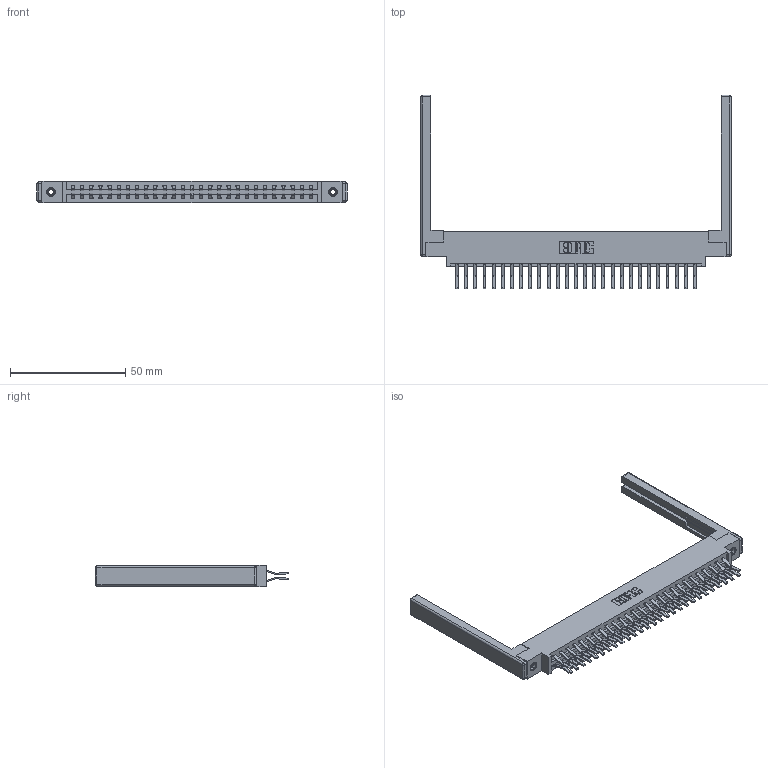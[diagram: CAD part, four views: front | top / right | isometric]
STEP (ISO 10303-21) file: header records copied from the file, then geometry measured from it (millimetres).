
FILE_DESCRIPTION (( 'STEP AP203' ), '1' );
FILE_NAME ('337-054-560-868.STEP', '2019-10-11T19:28:18', ( '' ), ( '' ), 'SwSTEP 2.0', 'SolidWorks 2016', '' );
FILE_SCHEMA (( 'CONFIG_CONTROL_DESIGN' ));
Length unit declared in the file: inch
Products named in the file (5): 307-220-068; 345-250-001_345-250-001-102; 345-292-001_560 Tail; 337-054-560-868; 337 Part_0.170 Offset - 0.156 Dia-TI
Assembly tree (59 placements, depth 2):
  337-054-560-868
    337 Part_0.170 Offset - 0.156 Dia-TI
    345-292-001_560 Tail  x54
    345-250-001_345-250-001-102  x2
    307-220-068  x2
Bounding box: 134.42 x 83.84 x 9.4 mm (x, y, z)
Volume: 18587.5 mm3; surface area: 21077.1 mm2
Topology: 59 solids, 59 shells, 3296 faces, 9731 edges, 6394 vertices
Faces by surface type: plane 2214, cylinder 1058, cone 12, sphere 8, torus 4
Entity records: 25854 total; most frequent: CARTESIAN_POINT 4335, ORIENTED_EDGE 4260, DIRECTION 3788, EDGE_CURVE 2130, LINE 1948, VECTOR 1948, VERTEX_POINT 1410, AXIS2_PLACEMENT_3D 920
